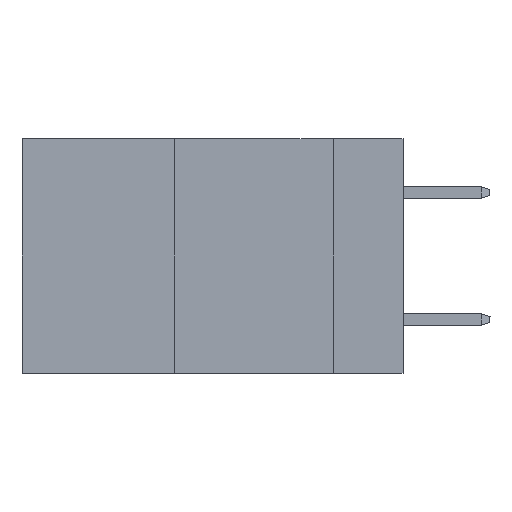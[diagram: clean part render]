
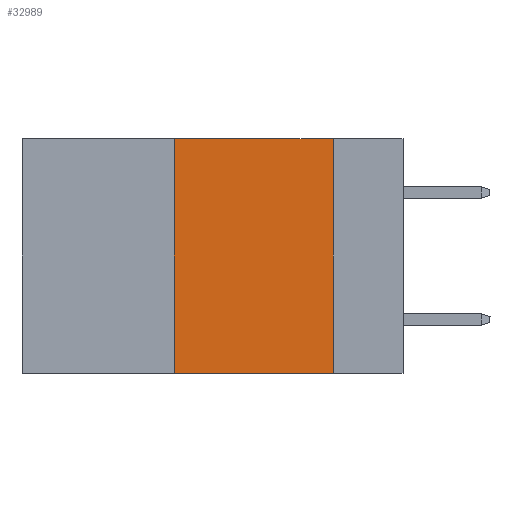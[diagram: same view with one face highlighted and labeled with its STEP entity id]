
A CAD part, left-side view. The second image highlights one B-rep face of the part: STEP entity #32989.
In plain terms, the highlighted planar face has unit normal (-1, 0, 0).
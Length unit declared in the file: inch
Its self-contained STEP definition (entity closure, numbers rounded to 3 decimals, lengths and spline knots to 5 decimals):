
#1560 = LINE ( 'NONE', #29347, #15076 ) ;
#2211 = CARTESIAN_POINT ( 'NONE',  ( 0., 0.11, 0. ) ) ;
#2502 = LINE ( 'NONE', #21890, #4691 ) ;
#4691 = VECTOR ( 'NONE', #25001, 39.37008 ) ;
#5139 = PLANE ( 'NONE',  #29062 ) ;
#7251 = CARTESIAN_POINT ( 'NONE',  ( 0., 0.6, 0. ) ) ;
#8024 = CARTESIAN_POINT ( 'NONE',  ( 0., 0.36, 0. ) ) ;
#9690 = DIRECTION ( 'NONE',  ( 0., 0., 1. ) ) ;
#11747 = CARTESIAN_POINT ( 'NONE',  ( 0., 0.11, -0.37 ) ) ;
#13511 = ORIENTED_EDGE ( 'NONE', *, *, #26573, .F. ) ;
#13597 = DIRECTION ( 'NONE',  ( 1., 0., 0. ) ) ;
#14874 = CARTESIAN_POINT ( 'NONE',  ( 0., 0.6, -0.37 ) ) ;
#15076 = VECTOR ( 'NONE', #9690, 39.37008 ) ;
#15153 = LINE ( 'NONE', #7251, #31201 ) ;
#15314 = VERTEX_POINT ( 'NONE', #8024 ) ;
#17282 = DIRECTION ( 'NONE',  ( 0., -1., 0. ) ) ;
#18773 = VERTEX_POINT ( 'NONE', #11747 ) ;
#20022 = ORIENTED_EDGE ( 'NONE', *, *, #23624, .T. ) ;
#21174 = CARTESIAN_POINT ( 'NONE',  ( 0., 0.36, -0.37 ) ) ;
#21890 = CARTESIAN_POINT ( 'NONE',  ( 0., 0.11, 0. ) ) ;
#21914 = CARTESIAN_POINT ( 'NONE',  ( 0., 0.6, 0. ) ) ;
#22038 = VERTEX_POINT ( 'NONE', #21174 ) ;
#22667 = ORIENTED_EDGE ( 'NONE', *, *, #25945, .F. ) ;
#22827 = EDGE_CURVE ( 'NONE', #22038, #15314, #1560, .T. ) ;
#23624 = EDGE_CURVE ( 'NONE', #22038, #18773, #28872, .T. ) ;
#23856 = EDGE_LOOP ( 'NONE', ( #22667, #13511, #33251, #20022 ) ) ;
#24837 = DIRECTION ( 'NONE',  ( 0., 0., -1. ) ) ;
#25001 = DIRECTION ( 'NONE',  ( 0., 0., -1. ) ) ;
#25531 = VERTEX_POINT ( 'NONE', #2211 ) ;
#25945 = EDGE_CURVE ( 'NONE', #25531, #18773, #2502, .T. ) ;
#26573 = EDGE_CURVE ( 'NONE', #15314, #25531, #15153, .T. ) ;
#28872 = LINE ( 'NONE', #14874, #33356 ) ;
#29062 = AXIS2_PLACEMENT_3D ( 'NONE', #21914, #13597, #24837 ) ;
#29347 = CARTESIAN_POINT ( 'NONE',  ( 0., 0.36, 0. ) ) ;
#30362 = FACE_OUTER_BOUND ( 'NONE', #23856, .T. ) ;
#31201 = VECTOR ( 'NONE', #35630, 39.37008 ) ;
#32989 = ADVANCED_FACE ( 'NONE', ( #30362 ), #5139, .F. ) ;
#33251 = ORIENTED_EDGE ( 'NONE', *, *, #22827, .F. ) ;
#33356 = VECTOR ( 'NONE', #17282, 39.37008 ) ;
#35630 = DIRECTION ( 'NONE',  ( 0., -1., 0. ) ) ;
